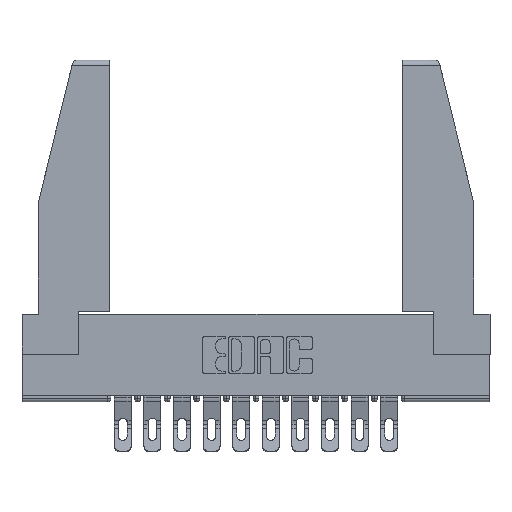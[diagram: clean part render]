
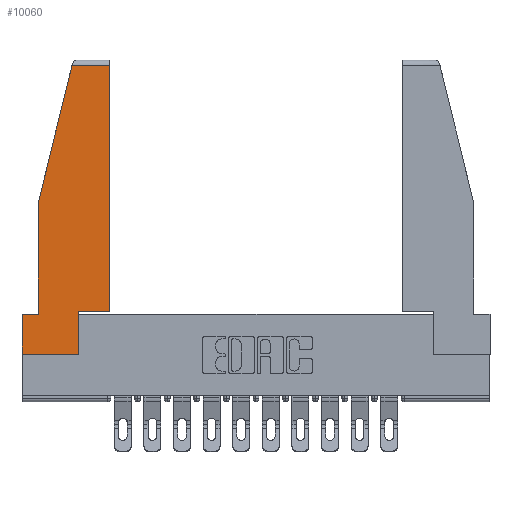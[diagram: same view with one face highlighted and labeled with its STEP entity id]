
A CAD part, top view. The second image highlights one B-rep face of the part: STEP entity #10060.
In plain terms, the highlighted planar face has unit normal (0, 0, 1).
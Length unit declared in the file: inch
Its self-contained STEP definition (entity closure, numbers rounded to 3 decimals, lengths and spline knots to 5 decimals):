
#153 = ORIENTED_EDGE ( 'NONE', *, *, #5719, .T. ) ;
#192 = ORIENTED_EDGE ( 'NONE', *, *, #12141, .T. ) ;
#217 = DIRECTION ( 'NONE',  ( 1., 0., 0. ) ) ;
#242 = CARTESIAN_POINT ( 'NONE',  ( 0., 0., 0. ) ) ;
#256 = CARTESIAN_POINT ( 'NONE',  ( 0.461, 0.223, 0. ) ) ;
#434 = EDGE_CURVE ( 'NONE', #17631, #12406, #6607, .T. ) ;
#851 = LINE ( 'NONE', #9878, #9692 ) ;
#917 = VECTOR ( 'NONE', #12022, 39.37008 ) ;
#1413 = EDGE_CURVE ( 'NONE', #7610, #9829, #16213, .T. ) ;
#1661 = VECTOR ( 'NONE', #8409, 39.37008 ) ;
#1779 = VERTEX_POINT ( 'NONE', #4283 ) ;
#1816 = DIRECTION ( 'NONE',  ( -1., 0., 0. ) ) ;
#3018 = DIRECTION ( 'NONE',  ( 0., -1., 0. ) ) ;
#3036 = CARTESIAN_POINT ( 'NONE',  ( 0., 0.21, 0. ) ) ;
#3099 = CARTESIAN_POINT ( 'NONE',  ( 0.086, 0.8, 0. ) ) ;
#3120 = DIRECTION ( 'NONE',  ( -0.239, -0.971, 0. ) ) ;
#3124 = AXIS2_PLACEMENT_3D ( 'NONE', #14649, #15861, #17221 ) ;
#3209 = EDGE_CURVE ( 'NONE', #16824, #17631, #851, .T. ) ;
#3557 = EDGE_CURVE ( 'NONE', #1779, #4169, #13982, .T. ) ;
#3880 = VECTOR ( 'NONE', #17716, 39.37008 ) ;
#4086 = LINE ( 'NONE', #16235, #3880 ) ;
#4169 = VERTEX_POINT ( 'NONE', #256 ) ;
#4283 = CARTESIAN_POINT ( 'NONE',  ( 0.297, 0.223, 0. ) ) ;
#4411 = CARTESIAN_POINT ( 'NONE',  ( 0.2636, 1.52, 0. ) ) ;
#5576 = CARTESIAN_POINT ( 'NONE',  ( 0.297, 0., 0. ) ) ;
#5658 = CARTESIAN_POINT ( 'NONE',  ( 0.461, 1.52, 0. ) ) ;
#5696 = EDGE_CURVE ( 'NONE', #9829, #13945, #16066, .T. ) ;
#5719 = EDGE_CURVE ( 'NONE', #13945, #8826, #10479, .T. ) ;
#5837 = ORIENTED_EDGE ( 'NONE', *, *, #3557, .T. ) ;
#5912 = CARTESIAN_POINT ( 'NONE',  ( 0.086, 0.21, 0. ) ) ;
#6607 = LINE ( 'NONE', #242, #13472 ) ;
#7454 = ORIENTED_EDGE ( 'NONE', *, *, #5696, .T. ) ;
#7610 = VERTEX_POINT ( 'NONE', #5658 ) ;
#7909 = FACE_OUTER_BOUND ( 'NONE', #13062, .T. ) ;
#8409 = DIRECTION ( 'NONE',  ( 0., -1., 0. ) ) ;
#8671 = EDGE_CURVE ( 'NONE', #12406, #1779, #4086, .T. ) ;
#8691 = LINE ( 'NONE', #12081, #917 ) ;
#8826 = VERTEX_POINT ( 'NONE', #5912 ) ;
#9121 = DIRECTION ( 'NONE',  ( 0., 1., 0. ) ) ;
#9692 = VECTOR ( 'NONE', #3018, 39.37008 ) ;
#9815 = ORIENTED_EDGE ( 'NONE', *, *, #8671, .T. ) ;
#9829 = VERTEX_POINT ( 'NONE', #4411 ) ;
#9878 = CARTESIAN_POINT ( 'NONE',  ( 0., 0.21, 0. ) ) ;
#10060 = ADVANCED_FACE ( 'NONE', ( #7909 ), #13096, .T. ) ;
#10078 = CARTESIAN_POINT ( 'NONE',  ( 0., 1.52, 0. ) ) ;
#10104 = ORIENTED_EDGE ( 'NONE', *, *, #434, .T. ) ;
#10173 = DIRECTION ( 'NONE',  ( 1., 0., 0. ) ) ;
#10323 = VECTOR ( 'NONE', #217, 39.37008 ) ;
#10479 = LINE ( 'NONE', #16625, #1661 ) ;
#11781 = VECTOR ( 'NONE', #3120, 39.37008 ) ;
#12022 = DIRECTION ( 'NONE',  ( -1., 0., 0. ) ) ;
#12081 = CARTESIAN_POINT ( 'NONE',  ( 0., 0.21, 0. ) ) ;
#12141 = EDGE_CURVE ( 'NONE', #8826, #16824, #8691, .T. ) ;
#12406 = VERTEX_POINT ( 'NONE', #5576 ) ;
#12440 = CARTESIAN_POINT ( 'NONE',  ( 0.271, 1.55, 0. ) ) ;
#12629 = CARTESIAN_POINT ( 'NONE',  ( 0., 0., 0. ) ) ;
#12938 = ORIENTED_EDGE ( 'NONE', *, *, #1413, .T. ) ;
#13062 = EDGE_LOOP ( 'NONE', ( #14155, #12938, #7454, #153, #192, #16725, #10104, #9815, #5837 ) ) ;
#13096 = PLANE ( 'NONE',  #3124 ) ;
#13132 = CARTESIAN_POINT ( 'NONE',  ( 0.461, 0.223, 0. ) ) ;
#13472 = VECTOR ( 'NONE', #10173, 39.37008 ) ;
#13628 = VECTOR ( 'NONE', #1816, 39.37008 ) ;
#13945 = VERTEX_POINT ( 'NONE', #3099 ) ;
#13982 = LINE ( 'NONE', #14774, #10323 ) ;
#14155 = ORIENTED_EDGE ( 'NONE', *, *, #14412, .T. ) ;
#14412 = EDGE_CURVE ( 'NONE', #4169, #7610, #14969, .T. ) ;
#14649 = CARTESIAN_POINT ( 'NONE',  ( 0., 0., 0. ) ) ;
#14774 = CARTESIAN_POINT ( 'NONE',  ( 0.297, 0.223, 0. ) ) ;
#14969 = LINE ( 'NONE', #13132, #15397 ) ;
#15397 = VECTOR ( 'NONE', #9121, 39.37008 ) ;
#15861 = DIRECTION ( 'NONE',  ( 0., 0., 1. ) ) ;
#16066 = LINE ( 'NONE', #12440, #11781 ) ;
#16213 = LINE ( 'NONE', #10078, #13628 ) ;
#16235 = CARTESIAN_POINT ( 'NONE',  ( 0.297, 0., 0. ) ) ;
#16625 = CARTESIAN_POINT ( 'NONE',  ( 0.086, 0.8, 0. ) ) ;
#16725 = ORIENTED_EDGE ( 'NONE', *, *, #3209, .T. ) ;
#16824 = VERTEX_POINT ( 'NONE', #3036 ) ;
#17221 = DIRECTION ( 'NONE',  ( 1., 0., 0. ) ) ;
#17631 = VERTEX_POINT ( 'NONE', #12629 ) ;
#17716 = DIRECTION ( 'NONE',  ( 0., 1., 0. ) ) ;
